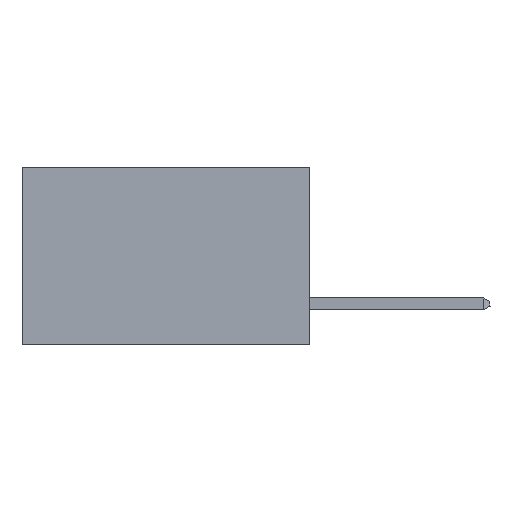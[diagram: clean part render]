
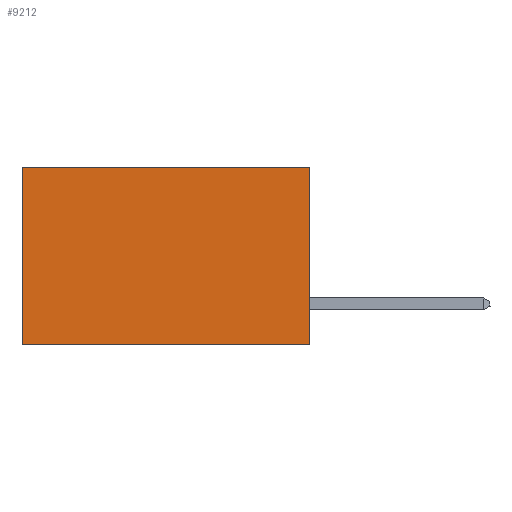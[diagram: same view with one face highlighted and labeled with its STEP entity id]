
A CAD part, left-side view. The second image highlights one B-rep face of the part: STEP entity #9212.
In plain terms, the highlighted planar face has unit normal (-1, 0, 0).
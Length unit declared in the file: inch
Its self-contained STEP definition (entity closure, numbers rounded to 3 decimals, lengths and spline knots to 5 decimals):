
#149 = DIRECTION ( 'NONE',  ( 1., 0., 0. ) ) ;
#251 = VECTOR ( 'NONE', #706, 39.37008 ) ;
#445 = LINE ( 'NONE', #3051, #7605 ) ;
#706 = DIRECTION ( 'NONE',  ( 0., 0., -1. ) ) ;
#818 = DIRECTION ( 'NONE',  ( 0., 1., 0. ) ) ;
#869 = PLANE ( 'NONE',  #7228 ) ;
#1268 = ORIENTED_EDGE ( 'NONE', *, *, #8346, .F. ) ;
#2566 = CARTESIAN_POINT ( 'NONE',  ( 0.2875, 0., 0. ) ) ;
#2578 = VECTOR ( 'NONE', #818, 39.37008 ) ;
#2770 = EDGE_CURVE ( 'NONE', #4400, #5546, #5157, .T. ) ;
#3024 = VERTEX_POINT ( 'NONE', #3180 ) ;
#3051 = CARTESIAN_POINT ( 'NONE',  ( 0.2875, 0., 0. ) ) ;
#3147 = CARTESIAN_POINT ( 'NONE',  ( 0.2875, 0., 0. ) ) ;
#3164 = CARTESIAN_POINT ( 'NONE',  ( 0.2875, 0., -0.37 ) ) ;
#3180 = CARTESIAN_POINT ( 'NONE',  ( 0.2875, 0., -0.37 ) ) ;
#3239 = FACE_OUTER_BOUND ( 'NONE', #9503, .T. ) ;
#3675 = CARTESIAN_POINT ( 'NONE',  ( 0.2875, 0.6, 0. ) ) ;
#3694 = ORIENTED_EDGE ( 'NONE', *, *, #5797, .T. ) ;
#3897 = CARTESIAN_POINT ( 'NONE',  ( 0.2875, 0.6, -0.37 ) ) ;
#4284 = LINE ( 'NONE', #3164, #2578 ) ;
#4400 = VERTEX_POINT ( 'NONE', #3675 ) ;
#4423 = EDGE_CURVE ( 'NONE', #3024, #5546, #4284, .T. ) ;
#4463 = CARTESIAN_POINT ( 'NONE',  ( 0.2875, 0.6, 0. ) ) ;
#4507 = DIRECTION ( 'NONE',  ( 0., 1., 0. ) ) ;
#4659 = ORIENTED_EDGE ( 'NONE', *, *, #2770, .T. ) ;
#4963 = LINE ( 'NONE', #5007, #6592 ) ;
#5007 = CARTESIAN_POINT ( 'NONE',  ( 0.2875, 0., 0. ) ) ;
#5157 = LINE ( 'NONE', #4463, #251 ) ;
#5546 = VERTEX_POINT ( 'NONE', #3897 ) ;
#5668 = DIRECTION ( 'NONE',  ( 0., 0., -1. ) ) ;
#5797 = EDGE_CURVE ( 'NONE', #6256, #4400, #445, .T. ) ;
#6256 = VERTEX_POINT ( 'NONE', #2566 ) ;
#6592 = VECTOR ( 'NONE', #5668, 39.37008 ) ;
#7228 = AXIS2_PLACEMENT_3D ( 'NONE', #3147, #149, #9187 ) ;
#7605 = VECTOR ( 'NONE', #4507, 39.37008 ) ;
#8053 = ORIENTED_EDGE ( 'NONE', *, *, #4423, .F. ) ;
#8346 = EDGE_CURVE ( 'NONE', #6256, #3024, #4963, .T. ) ;
#9187 = DIRECTION ( 'NONE',  ( 0., 0., -1. ) ) ;
#9212 = ADVANCED_FACE ( 'NONE', ( #3239 ), #869, .F. ) ;
#9503 = EDGE_LOOP ( 'NONE', ( #4659, #8053, #1268, #3694 ) ) ;
